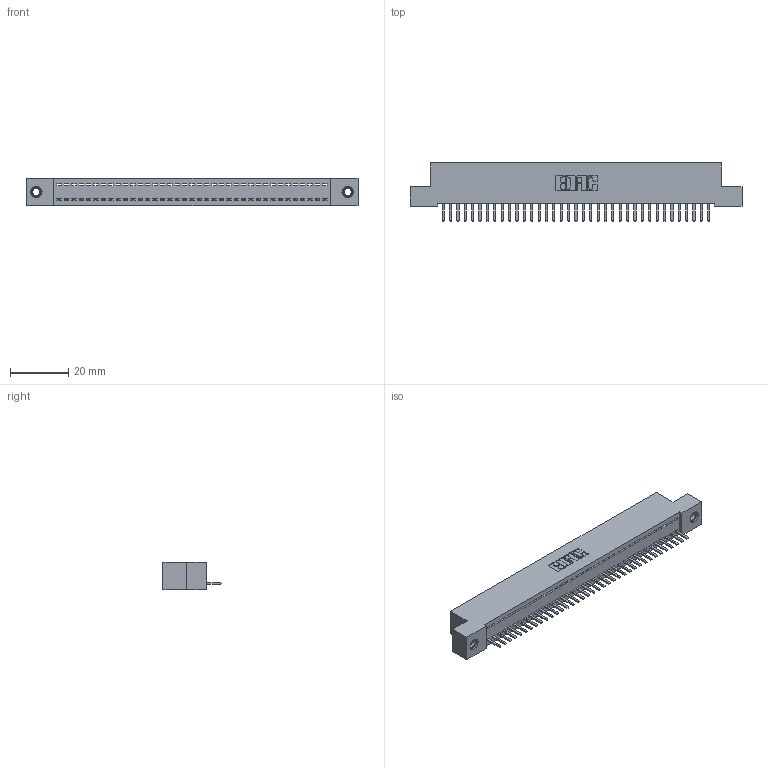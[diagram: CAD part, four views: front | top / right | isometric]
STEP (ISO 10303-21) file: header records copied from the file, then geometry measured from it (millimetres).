
FILE_DESCRIPTION (( 'STEP AP203' ), '1' );
FILE_NAME ('392-037-520-107.STEP', '2018-08-16T04:11:01', ( '' ), ( '' ), 'SwSTEP 2.0', 'SolidWorks 2016', '' );
FILE_SCHEMA (( 'CONFIG_CONTROL_DESIGN' ));
Length unit declared in the file: inch
Products named in the file (4): 342 Part_TI; 345-292-001_345-293-120; 345-250-001_345-250-005-103; 392-037-520-107
Assembly tree (40 placements, depth 2):
  392-037-520-107
    342 Part_TI
    345-292-001_345-293-120  x37
    345-250-001_345-250-005-103  x2
Bounding box: 114.3 x 20.02 x 9.4 mm (x, y, z)
Volume: 9884.3 mm3; surface area: 14113.1 mm2
Topology: 40 solids, 40 shells, 2464 faces, 7243 edges, 4722 vertices
Faces by surface type: plane 1726, cylinder 722, cone 12, torus 4
Entity records: 24434 total; most frequent: CARTESIAN_POINT 4208, ORIENTED_EDGE 4162, DIRECTION 3581, EDGE_CURVE 2081, VECTOR 1929, LINE 1929, VERTEX_POINT 1380, AXIS2_PLACEMENT_3D 826
